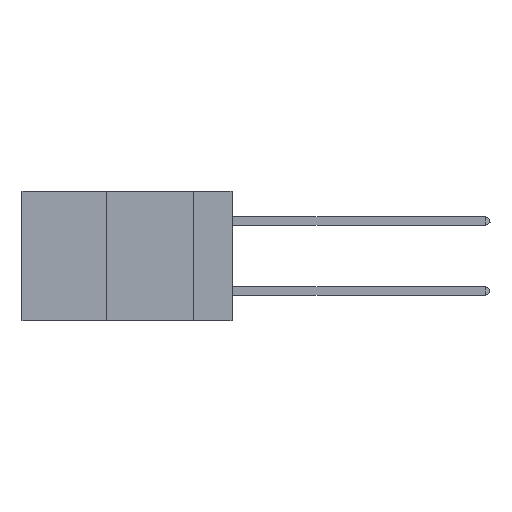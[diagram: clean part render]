
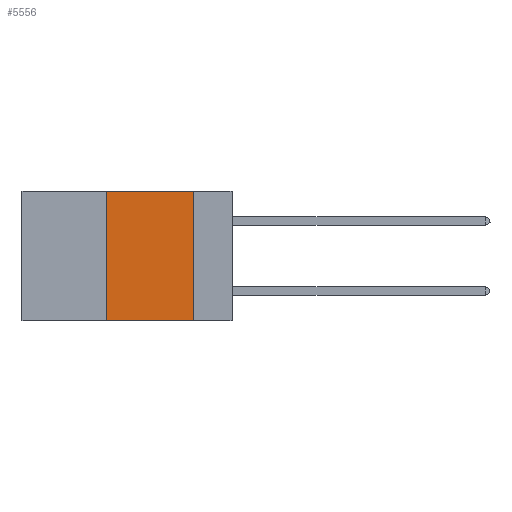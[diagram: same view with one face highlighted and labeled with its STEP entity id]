
A CAD part, left-side view. The second image highlights one B-rep face of the part: STEP entity #5556.
In plain terms, the highlighted planar face has unit normal (-1, 0, 0).
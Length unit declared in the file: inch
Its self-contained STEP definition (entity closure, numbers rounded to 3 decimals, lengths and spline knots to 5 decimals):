
#250 = AXIS2_PLACEMENT_3D ( 'NONE', #16245, #19669, #7921 ) ;
#749 = CARTESIAN_POINT ( 'NONE',  ( 0., 0.11, -0.37 ) ) ;
#1189 = CARTESIAN_POINT ( 'NONE',  ( 0., 0.6, -0.37 ) ) ;
#1320 = EDGE_LOOP ( 'NONE', ( #15230, #20469, #19780, #12451 ) ) ;
#3316 = CARTESIAN_POINT ( 'NONE',  ( 0., 0.11, 0. ) ) ;
#3882 = EDGE_CURVE ( 'NONE', #5814, #9539, #13559, .T. ) ;
#4239 = DIRECTION ( 'NONE',  ( 0., -1., 0. ) ) ;
#4509 = LINE ( 'NONE', #1189, #9177 ) ;
#5556 = ADVANCED_FACE ( 'NONE', ( #14249 ), #7591, .F. ) ;
#5607 = VERTEX_POINT ( 'NONE', #749 ) ;
#5814 = VERTEX_POINT ( 'NONE', #15025 ) ;
#6653 = LINE ( 'NONE', #3316, #13248 ) ;
#6683 = EDGE_CURVE ( 'NONE', #13454, #5607, #6653, .T. ) ;
#7591 = PLANE ( 'NONE',  #250 ) ;
#7921 = DIRECTION ( 'NONE',  ( 0., 0., -1. ) ) ;
#8155 = VECTOR ( 'NONE', #4239, 39.37008 ) ;
#8190 = EDGE_CURVE ( 'NONE', #5814, #5607, #4509, .T. ) ;
#8559 = DIRECTION ( 'NONE',  ( 0., 0., 1. ) ) ;
#9177 = VECTOR ( 'NONE', #14583, 39.37008 ) ;
#9539 = VERTEX_POINT ( 'NONE', #12964 ) ;
#10826 = EDGE_CURVE ( 'NONE', #9539, #13454, #17438, .T. ) ;
#10990 = CARTESIAN_POINT ( 'NONE',  ( 0., 0.6, 0. ) ) ;
#11845 = DIRECTION ( 'NONE',  ( 0., 0., -1. ) ) ;
#11996 = CARTESIAN_POINT ( 'NONE',  ( 0., 0.36, 0. ) ) ;
#12451 = ORIENTED_EDGE ( 'NONE', *, *, #8190, .T. ) ;
#12964 = CARTESIAN_POINT ( 'NONE',  ( 0., 0.36, 0. ) ) ;
#13248 = VECTOR ( 'NONE', #11845, 39.37008 ) ;
#13454 = VERTEX_POINT ( 'NONE', #17642 ) ;
#13559 = LINE ( 'NONE', #11996, #21642 ) ;
#14249 = FACE_OUTER_BOUND ( 'NONE', #1320, .T. ) ;
#14583 = DIRECTION ( 'NONE',  ( 0., -1., 0. ) ) ;
#15025 = CARTESIAN_POINT ( 'NONE',  ( 0., 0.36, -0.37 ) ) ;
#15230 = ORIENTED_EDGE ( 'NONE', *, *, #6683, .F. ) ;
#16245 = CARTESIAN_POINT ( 'NONE',  ( 0., 0.6, 0. ) ) ;
#17438 = LINE ( 'NONE', #10990, #8155 ) ;
#17642 = CARTESIAN_POINT ( 'NONE',  ( 0., 0.11, 0. ) ) ;
#19669 = DIRECTION ( 'NONE',  ( 1., 0., 0. ) ) ;
#19780 = ORIENTED_EDGE ( 'NONE', *, *, #3882, .F. ) ;
#20469 = ORIENTED_EDGE ( 'NONE', *, *, #10826, .F. ) ;
#21642 = VECTOR ( 'NONE', #8559, 39.37008 ) ;
